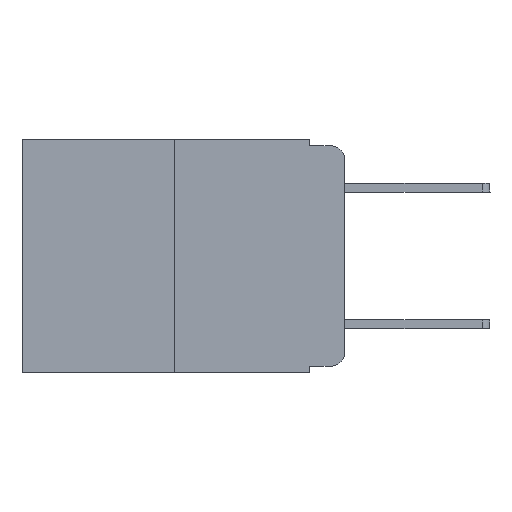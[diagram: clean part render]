
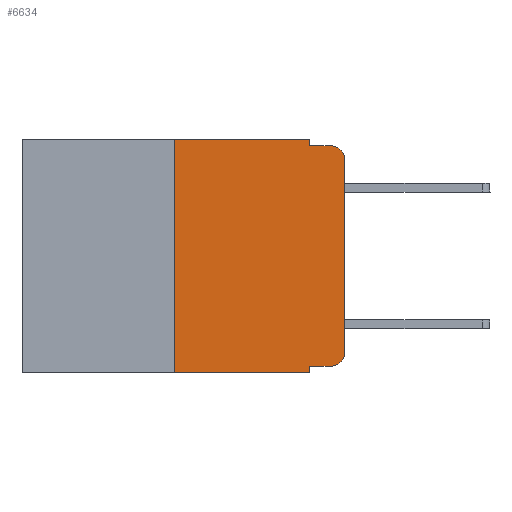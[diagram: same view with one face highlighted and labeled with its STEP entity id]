
A CAD part, left-side view. The second image highlights one B-rep face of the part: STEP entity #6634.
In plain terms, the highlighted planar face has unit normal (-1, 0, 0).
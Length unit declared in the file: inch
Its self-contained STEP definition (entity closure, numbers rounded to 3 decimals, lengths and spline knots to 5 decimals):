
#19 = AXIS2_PLACEMENT_3D ( 'NONE', #254, #5724, #1819 ) ;
#210 = EDGE_CURVE ( 'NONE', #264, #8168, #9104, .T. ) ;
#226 = DIRECTION ( 'NONE',  ( 0., 0., -1. ) ) ;
#254 = CARTESIAN_POINT ( 'NONE',  ( 0., 0.473, 0. ) ) ;
#256 = EDGE_LOOP ( 'NONE', ( #9259, #6590, #7018, #985, #2534, #6398, #7645, #1270, #3642, #5247 ) ) ;
#264 = VERTEX_POINT ( 'NONE', #7639 ) ;
#287 = EDGE_CURVE ( 'NONE', #9596, #1772, #5674, .T. ) ;
#290 = VECTOR ( 'NONE', #9279, 39.37008 ) ;
#430 = DIRECTION ( 'NONE',  ( 0., -1., 0. ) ) ;
#621 = EDGE_CURVE ( 'NONE', #9058, #6267, #4789, .T. ) ;
#741 = EDGE_CURVE ( 'NONE', #2572, #8168, #4908, .T. ) ;
#883 = DIRECTION ( 'NONE',  ( 0., -1., 0. ) ) ;
#985 = ORIENTED_EDGE ( 'NONE', *, *, #7098, .F. ) ;
#1270 = ORIENTED_EDGE ( 'NONE', *, *, #741, .F. ) ;
#1310 = CARTESIAN_POINT ( 'NONE',  ( 0., 0.02, -0.333 ) ) ;
#1373 = VECTOR ( 'NONE', #226, 39.37008 ) ;
#1501 = DIRECTION ( 'NONE',  ( 0., 0., -1. ) ) ;
#1772 = VERTEX_POINT ( 'NONE', #9754 ) ;
#1819 = DIRECTION ( 'NONE',  ( 0., 0., -1. ) ) ;
#1894 = LINE ( 'NONE', #6188, #9884 ) ;
#1936 = LINE ( 'NONE', #8877, #3037 ) ;
#2070 = DIRECTION ( 'NONE',  ( 0., 0., -1. ) ) ;
#2134 = CIRCLE ( 'NONE', #8517, 0.02 ) ;
#2307 = DIRECTION ( 'NONE',  ( 0., 0., -1. ) ) ;
#2534 = ORIENTED_EDGE ( 'NONE', *, *, #621, .F. ) ;
#2572 = VERTEX_POINT ( 'NONE', #7393 ) ;
#2658 = CARTESIAN_POINT ( 'NONE',  ( 0., 0.051, -0.333 ) ) ;
#2764 = DIRECTION ( 'NONE',  ( 0., -1., 0. ) ) ;
#3037 = VECTOR ( 'NONE', #5241, 39.37008 ) ;
#3149 = CARTESIAN_POINT ( 'NONE',  ( 0., 0.051, 0. ) ) ;
#3163 = EDGE_CURVE ( 'NONE', #9687, #3508, #5240, .T. ) ;
#3508 = VERTEX_POINT ( 'NONE', #4995 ) ;
#3642 = ORIENTED_EDGE ( 'NONE', *, *, #7950, .T. ) ;
#3648 = VERTEX_POINT ( 'NONE', #5412 ) ;
#3677 = CARTESIAN_POINT ( 'NONE',  ( 0., 0.25, 0. ) ) ;
#3702 = VECTOR ( 'NONE', #2307, 39.37008 ) ;
#3847 = DIRECTION ( 'NONE',  ( -1., 0., 0. ) ) ;
#3865 = AXIS2_PLACEMENT_3D ( 'NONE', #8449, #3847, #1501 ) ;
#4789 = LINE ( 'NONE', #5883, #7382 ) ;
#4908 = LINE ( 'NONE', #5767, #1373 ) ;
#4923 = PLANE ( 'NONE',  #19 ) ;
#4995 = CARTESIAN_POINT ( 'NONE',  ( 0., 0.02, -0.01 ) ) ;
#5173 = DIRECTION ( 'NONE',  ( -1., 0., 0. ) ) ;
#5240 = LINE ( 'NONE', #5533, #7814 ) ;
#5241 = DIRECTION ( 'NONE',  ( 0., 0., 1. ) ) ;
#5247 = ORIENTED_EDGE ( 'NONE', *, *, #287, .T. ) ;
#5408 = EDGE_CURVE ( 'NONE', #264, #9058, #1894, .T. ) ;
#5412 = CARTESIAN_POINT ( 'NONE',  ( 0., 0., -0.03 ) ) ;
#5533 = CARTESIAN_POINT ( 'NONE',  ( 0., 0.051, -0.01 ) ) ;
#5674 = CIRCLE ( 'NONE', #3865, 0.02 ) ;
#5724 = DIRECTION ( 'NONE',  ( 1., 0., 0. ) ) ;
#5767 = CARTESIAN_POINT ( 'NONE',  ( 0., 0.051, 0. ) ) ;
#5883 = CARTESIAN_POINT ( 'NONE',  ( 0., 0.473, 0. ) ) ;
#6188 = CARTESIAN_POINT ( 'NONE',  ( 0., 0.25, 0. ) ) ;
#6230 = EDGE_CURVE ( 'NONE', #3648, #3508, #2134, .T. ) ;
#6267 = VERTEX_POINT ( 'NONE', #7514 ) ;
#6398 = ORIENTED_EDGE ( 'NONE', *, *, #5408, .F. ) ;
#6590 = ORIENTED_EDGE ( 'NONE', *, *, #6230, .T. ) ;
#6592 = CARTESIAN_POINT ( 'NONE',  ( 0., 0.473, -0.343 ) ) ;
#6634 = ADVANCED_FACE ( 'NONE', ( #7025 ), #4923, .F. ) ;
#7018 = ORIENTED_EDGE ( 'NONE', *, *, #3163, .F. ) ;
#7025 = FACE_OUTER_BOUND ( 'NONE', #256, .T. ) ;
#7063 = CARTESIAN_POINT ( 'NONE',  ( 0., 0.051, -0.343 ) ) ;
#7098 = EDGE_CURVE ( 'NONE', #6267, #9687, #9983, .T. ) ;
#7382 = VECTOR ( 'NONE', #2764, 39.37008 ) ;
#7393 = CARTESIAN_POINT ( 'NONE',  ( 0., 0.051, -0.333 ) ) ;
#7514 = CARTESIAN_POINT ( 'NONE',  ( 0., 0.051, 0. ) ) ;
#7542 = CARTESIAN_POINT ( 'NONE',  ( 0., 0.051, -0.01 ) ) ;
#7585 = CARTESIAN_POINT ( 'NONE',  ( 0., 0.02, -0.03 ) ) ;
#7639 = CARTESIAN_POINT ( 'NONE',  ( 0., 0.25, -0.343 ) ) ;
#7645 = ORIENTED_EDGE ( 'NONE', *, *, #210, .T. ) ;
#7814 = VECTOR ( 'NONE', #883, 39.37008 ) ;
#7950 = EDGE_CURVE ( 'NONE', #2572, #9596, #9834, .T. ) ;
#8168 = VERTEX_POINT ( 'NONE', #7063 ) ;
#8449 = CARTESIAN_POINT ( 'NONE',  ( 0., 0.02, -0.313 ) ) ;
#8517 = AXIS2_PLACEMENT_3D ( 'NONE', #7585, #5173, #2070 ) ;
#8708 = VECTOR ( 'NONE', #430, 39.37008 ) ;
#8877 = CARTESIAN_POINT ( 'NONE',  ( 0., 0., 0. ) ) ;
#9058 = VERTEX_POINT ( 'NONE', #3677 ) ;
#9104 = LINE ( 'NONE', #6592, #290 ) ;
#9229 = DIRECTION ( 'NONE',  ( 0., 0., 1. ) ) ;
#9259 = ORIENTED_EDGE ( 'NONE', *, *, #9595, .T. ) ;
#9279 = DIRECTION ( 'NONE',  ( 0., -1., 0. ) ) ;
#9595 = EDGE_CURVE ( 'NONE', #1772, #3648, #1936, .T. ) ;
#9596 = VERTEX_POINT ( 'NONE', #1310 ) ;
#9687 = VERTEX_POINT ( 'NONE', #7542 ) ;
#9754 = CARTESIAN_POINT ( 'NONE',  ( 0., 0., -0.313 ) ) ;
#9834 = LINE ( 'NONE', #2658, #8708 ) ;
#9884 = VECTOR ( 'NONE', #9229, 39.37008 ) ;
#9983 = LINE ( 'NONE', #3149, #3702 ) ;
